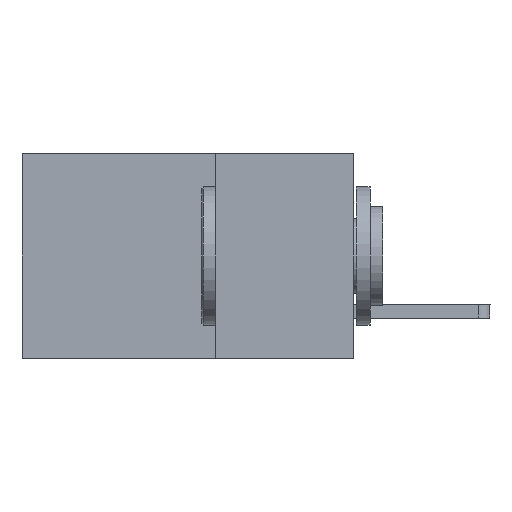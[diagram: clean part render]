
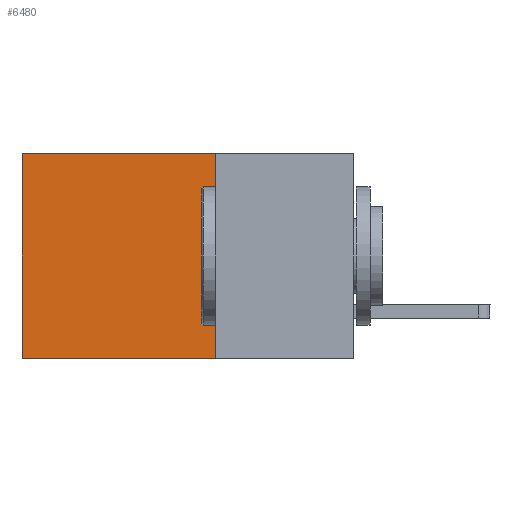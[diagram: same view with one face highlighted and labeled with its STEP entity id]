
A CAD part, left-side view. The second image highlights one B-rep face of the part: STEP entity #6480.
In plain terms, the highlighted planar face has unit normal (-1, 0, 0).
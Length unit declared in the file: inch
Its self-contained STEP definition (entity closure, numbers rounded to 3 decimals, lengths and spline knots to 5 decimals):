
#109 = EDGE_CURVE ( 'NONE', #7815, #3671, #7471, .T. ) ;
#174 = DIRECTION ( 'NONE',  ( 0., 0., -1. ) ) ;
#214 = CARTESIAN_POINT ( 'NONE',  ( 0.2875, 0.25, 0. ) ) ;
#329 = EDGE_LOOP ( 'NONE', ( #9057, #4644, #11357, #651 ) ) ;
#637 = EDGE_CURVE ( 'NONE', #3671, #7075, #11815, .T. ) ;
#651 = ORIENTED_EDGE ( 'NONE', *, *, #7795, .T. ) ;
#874 = VECTOR ( 'NONE', #8010, 39.37008 ) ;
#1006 = VECTOR ( 'NONE', #10594, 39.37008 ) ;
#1863 = CARTESIAN_POINT ( 'NONE',  ( 0.2875, 0.25, 0. ) ) ;
#2081 = LINE ( 'NONE', #1863, #4962 ) ;
#2932 = CARTESIAN_POINT ( 'NONE',  ( 0.2875, 0.25, 0. ) ) ;
#3597 = CARTESIAN_POINT ( 'NONE',  ( 0.2875, 0.6, 0. ) ) ;
#3671 = VERTEX_POINT ( 'NONE', #6318 ) ;
#4361 = FACE_OUTER_BOUND ( 'NONE', #329, .T. ) ;
#4644 = ORIENTED_EDGE ( 'NONE', *, *, #637, .F. ) ;
#4962 = VECTOR ( 'NONE', #9462, 39.37008 ) ;
#5318 = CARTESIAN_POINT ( 'NONE',  ( 0.2875, 0.6, 0. ) ) ;
#5519 = DIRECTION ( 'NONE',  ( 0., 0., -1. ) ) ;
#5946 = PLANE ( 'NONE',  #10533 ) ;
#6318 = CARTESIAN_POINT ( 'NONE',  ( 0.2875, 0.25, -0.37 ) ) ;
#6480 = ADVANCED_FACE ( 'NONE', ( #4361 ), #5946, .F. ) ;
#6856 = DIRECTION ( 'NONE',  ( 1., 0., 0. ) ) ;
#7021 = VECTOR ( 'NONE', #5519, 39.37008 ) ;
#7075 = VERTEX_POINT ( 'NONE', #7463 ) ;
#7463 = CARTESIAN_POINT ( 'NONE',  ( 0.2875, 0.6, -0.37 ) ) ;
#7471 = LINE ( 'NONE', #214, #874 ) ;
#7795 = EDGE_CURVE ( 'NONE', #7815, #10159, #2081, .T. ) ;
#7815 = VERTEX_POINT ( 'NONE', #2932 ) ;
#7938 = CARTESIAN_POINT ( 'NONE',  ( 0.2875, 0.25, 0. ) ) ;
#8010 = DIRECTION ( 'NONE',  ( 0., 0., -1. ) ) ;
#8119 = EDGE_CURVE ( 'NONE', #10159, #7075, #9735, .T. ) ;
#9057 = ORIENTED_EDGE ( 'NONE', *, *, #8119, .T. ) ;
#9462 = DIRECTION ( 'NONE',  ( 0., 1., 0. ) ) ;
#9626 = CARTESIAN_POINT ( 'NONE',  ( 0.2875, 0.25, -0.37 ) ) ;
#9735 = LINE ( 'NONE', #3597, #7021 ) ;
#10159 = VERTEX_POINT ( 'NONE', #5318 ) ;
#10533 = AXIS2_PLACEMENT_3D ( 'NONE', #7938, #6856, #174 ) ;
#10594 = DIRECTION ( 'NONE',  ( 0., 1., 0. ) ) ;
#11357 = ORIENTED_EDGE ( 'NONE', *, *, #109, .F. ) ;
#11815 = LINE ( 'NONE', #9626, #1006 ) ;
